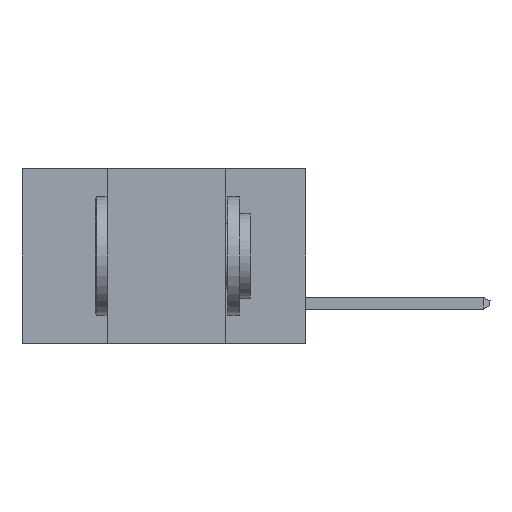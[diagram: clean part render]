
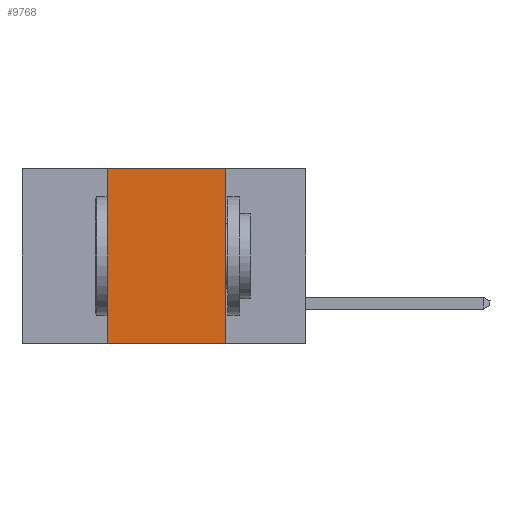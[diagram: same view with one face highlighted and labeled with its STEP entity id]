
A CAD part, left-side view. The second image highlights one B-rep face of the part: STEP entity #9768.
In plain terms, the highlighted planar face has unit normal (-1, 0, 0).
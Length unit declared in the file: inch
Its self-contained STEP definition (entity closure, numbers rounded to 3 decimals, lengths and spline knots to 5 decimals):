
#1263 = EDGE_CURVE ( 'NONE', #11021, #15589, #22764, .T. ) ;
#1512 = VERTEX_POINT ( 'NONE', #12041 ) ;
#2500 = VECTOR ( 'NONE', #21393, 39.37008 ) ;
#3862 = CARTESIAN_POINT ( 'NONE',  ( 0., 0.17, -0.37 ) ) ;
#4285 = FACE_OUTER_BOUND ( 'NONE', #20080, .T. ) ;
#4549 = DIRECTION ( 'NONE',  ( 0., 0., -1. ) ) ;
#4574 = DIRECTION ( 'NONE',  ( 1., 0., 0. ) ) ;
#4598 = PLANE ( 'NONE',  #23637 ) ;
#4680 = CARTESIAN_POINT ( 'NONE',  ( 0., 0.6, 0. ) ) ;
#7878 = VECTOR ( 'NONE', #23837, 39.37008 ) ;
#8679 = VECTOR ( 'NONE', #10360, 39.37008 ) ;
#9278 = LINE ( 'NONE', #9725, #8679 ) ;
#9725 = CARTESIAN_POINT ( 'NONE',  ( 0., 0.6, 0. ) ) ;
#9768 = ADVANCED_FACE ( 'NONE', ( #4285 ), #4598, .F. ) ;
#10360 = DIRECTION ( 'NONE',  ( 0., -1., 0. ) ) ;
#10588 = EDGE_CURVE ( 'NONE', #16061, #1512, #9278, .T. ) ;
#11021 = VERTEX_POINT ( 'NONE', #21974 ) ;
#11043 = DIRECTION ( 'NONE',  ( 0., 0., 1. ) ) ;
#11311 = CARTESIAN_POINT ( 'NONE',  ( 0., 0.42, -0.37 ) ) ;
#11969 = EDGE_CURVE ( 'NONE', #11021, #16061, #13107, .T. ) ;
#12041 = CARTESIAN_POINT ( 'NONE',  ( 0., 0.17, 0. ) ) ;
#13107 = LINE ( 'NONE', #11311, #17624 ) ;
#14333 = ORIENTED_EDGE ( 'NONE', *, *, #10588, .F. ) ;
#15589 = VERTEX_POINT ( 'NONE', #3862 ) ;
#16061 = VERTEX_POINT ( 'NONE', #19507 ) ;
#16739 = ORIENTED_EDGE ( 'NONE', *, *, #1263, .T. ) ;
#17624 = VECTOR ( 'NONE', #11043, 39.37008 ) ;
#17952 = ORIENTED_EDGE ( 'NONE', *, *, #11969, .F. ) ;
#19507 = CARTESIAN_POINT ( 'NONE',  ( 0., 0.42, 0. ) ) ;
#20080 = EDGE_LOOP ( 'NONE', ( #20585, #14333, #17952, #16739 ) ) ;
#20585 = ORIENTED_EDGE ( 'NONE', *, *, #20833, .F. ) ;
#20833 = EDGE_CURVE ( 'NONE', #1512, #15589, #23050, .T. ) ;
#21393 = DIRECTION ( 'NONE',  ( 0., -1., 0. ) ) ;
#21608 = CARTESIAN_POINT ( 'NONE',  ( 0., 0.6, -0.37 ) ) ;
#21974 = CARTESIAN_POINT ( 'NONE',  ( 0., 0.42, -0.37 ) ) ;
#22764 = LINE ( 'NONE', #21608, #2500 ) ;
#23050 = LINE ( 'NONE', #23766, #7878 ) ;
#23637 = AXIS2_PLACEMENT_3D ( 'NONE', #4680, #4574, #4549 ) ;
#23766 = CARTESIAN_POINT ( 'NONE',  ( 0., 0.17, -0.37 ) ) ;
#23837 = DIRECTION ( 'NONE',  ( 0., 0., -1. ) ) ;
